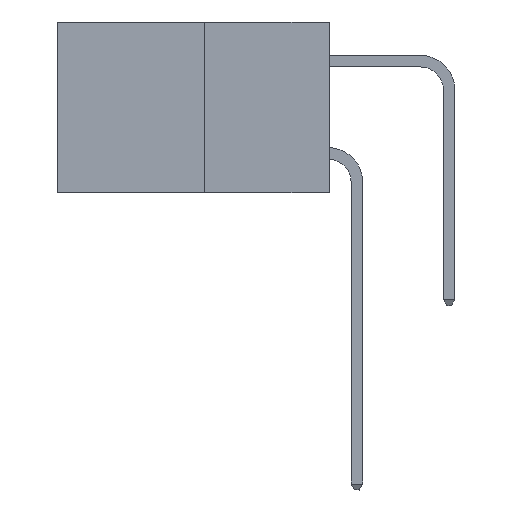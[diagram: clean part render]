
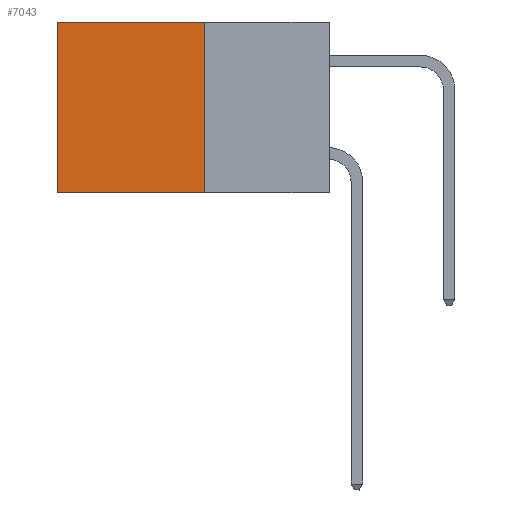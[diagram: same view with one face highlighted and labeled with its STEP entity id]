
A CAD part, left-side view. The second image highlights one B-rep face of the part: STEP entity #7043.
In plain terms, the highlighted planar face has unit normal (-1, 0, 0).
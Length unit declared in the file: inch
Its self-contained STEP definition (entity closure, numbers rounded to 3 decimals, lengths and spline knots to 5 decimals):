
#950 = LINE ( 'NONE', #19754, #15278 ) ;
#1219 = ORIENTED_EDGE ( 'NONE', *, *, #15742, .T. ) ;
#2915 = LINE ( 'NONE', #13587, #32159 ) ;
#3127 = FACE_OUTER_BOUND ( 'NONE', #20008, .T. ) ;
#5225 = DIRECTION ( 'NONE',  ( 0., 0., -1. ) ) ;
#5434 = CARTESIAN_POINT ( 'NONE',  ( 0.277, 0.27, -0.37 ) ) ;
#6234 = LINE ( 'NONE', #32472, #13003 ) ;
#6986 = CARTESIAN_POINT ( 'NONE',  ( 0.277, 0.59, 0. ) ) ;
#7043 = ADVANCED_FACE ( 'NONE', ( #3127 ), #35521, .F. ) ;
#7560 = AXIS2_PLACEMENT_3D ( 'NONE', #35322, #34919, #34879 ) ;
#7901 = EDGE_CURVE ( 'NONE', #14109, #25738, #20074, .T. ) ;
#12374 = EDGE_CURVE ( 'NONE', #25738, #14451, #2915, .T. ) ;
#12543 = VECTOR ( 'NONE', #5225, 39.37008 ) ;
#13003 = VECTOR ( 'NONE', #18537, 39.37008 ) ;
#13587 = CARTESIAN_POINT ( 'NONE',  ( 0.277, 0.27, -0.37 ) ) ;
#14109 = VERTEX_POINT ( 'NONE', #28906 ) ;
#14173 = DIRECTION ( 'NONE',  ( 0., 1., 0. ) ) ;
#14451 = VERTEX_POINT ( 'NONE', #25285 ) ;
#15278 = VECTOR ( 'NONE', #14173, 39.37008 ) ;
#15742 = EDGE_CURVE ( 'NONE', #14109, #16081, #950, .T. ) ;
#16081 = VERTEX_POINT ( 'NONE', #6986 ) ;
#18347 = EDGE_CURVE ( 'NONE', #16081, #14451, #6234, .T. ) ;
#18537 = DIRECTION ( 'NONE',  ( 0., 0., -1. ) ) ;
#19754 = CARTESIAN_POINT ( 'NONE',  ( 0.277, 0.27, 0. ) ) ;
#20008 = EDGE_LOOP ( 'NONE', ( #26456, #30630, #25028, #1219 ) ) ;
#20074 = LINE ( 'NONE', #5434, #12543 ) ;
#20356 = CARTESIAN_POINT ( 'NONE',  ( 0.277, 0.27, -0.37 ) ) ;
#25028 = ORIENTED_EDGE ( 'NONE', *, *, #7901, .F. ) ;
#25285 = CARTESIAN_POINT ( 'NONE',  ( 0.277, 0.59, -0.37 ) ) ;
#25738 = VERTEX_POINT ( 'NONE', #20356 ) ;
#26456 = ORIENTED_EDGE ( 'NONE', *, *, #18347, .T. ) ;
#28906 = CARTESIAN_POINT ( 'NONE',  ( 0.277, 0.27, 0. ) ) ;
#30445 = DIRECTION ( 'NONE',  ( 0., 1., 0. ) ) ;
#30630 = ORIENTED_EDGE ( 'NONE', *, *, #12374, .F. ) ;
#32159 = VECTOR ( 'NONE', #30445, 39.37008 ) ;
#32472 = CARTESIAN_POINT ( 'NONE',  ( 0.277, 0.59, -0.37 ) ) ;
#34879 = DIRECTION ( 'NONE',  ( 0., 0., -1. ) ) ;
#34919 = DIRECTION ( 'NONE',  ( 1., 0., 0. ) ) ;
#35322 = CARTESIAN_POINT ( 'NONE',  ( 0.277, 0.27, -0.37 ) ) ;
#35521 = PLANE ( 'NONE',  #7560 ) ;
